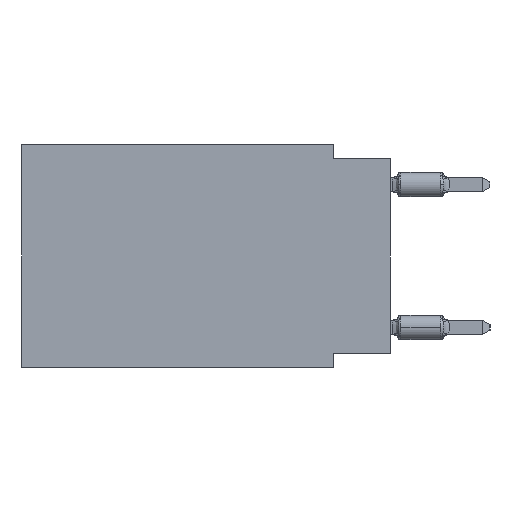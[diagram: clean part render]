
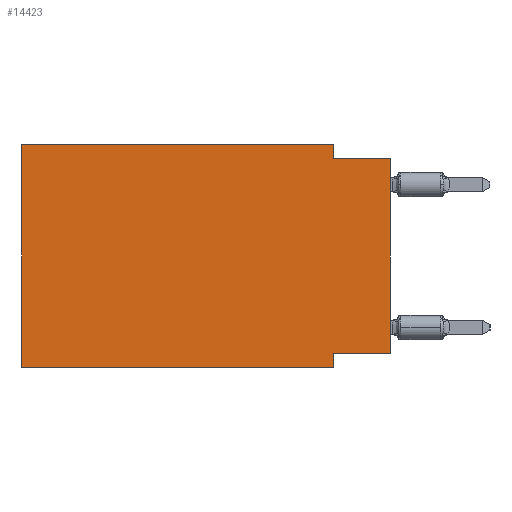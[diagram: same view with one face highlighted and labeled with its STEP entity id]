
A CAD part, left-side view. The second image highlights one B-rep face of the part: STEP entity #14423.
In plain terms, the highlighted planar face has unit normal (-1, 0, 0).
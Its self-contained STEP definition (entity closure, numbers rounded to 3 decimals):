
#656 = DIRECTION ( 'NONE',  ( 1., 0., 0. ) ) ;
#1021 = VERTEX_POINT ( 'NONE', #26408 ) ;
#1884 = DIRECTION ( 'NONE',  ( 0., -1., 0. ) ) ;
#2759 = VERTEX_POINT ( 'NONE', #11449 ) ;
#3206 = CARTESIAN_POINT ( 'NONE',  ( 0., 2.54, -9.271 ) ) ;
#4237 = ORIENTED_EDGE ( 'NONE', *, *, #25664, .F. ) ;
#4959 = VERTEX_POINT ( 'NONE', #14895 ) ;
#5066 = CARTESIAN_POINT ( 'NONE',  ( 0., 16.383, 0. ) ) ;
#6006 = DIRECTION ( 'NONE',  ( 0., 1., 0. ) ) ;
#6277 = CARTESIAN_POINT ( 'NONE',  ( 0., 2.54, -9.906 ) ) ;
#6389 = LINE ( 'NONE', #38236, #24654 ) ;
#6845 = VECTOR ( 'NONE', #6006, 1000. ) ;
#7046 = PLANE ( 'NONE',  #23246 ) ;
#7713 = DIRECTION ( 'NONE',  ( 0., 0., -1. ) ) ;
#7974 = DIRECTION ( 'NONE',  ( 0., -1., 0. ) ) ;
#8140 = VECTOR ( 'NONE', #1884, 1000. ) ;
#8549 = DIRECTION ( 'NONE',  ( 0., 0., 1. ) ) ;
#8664 = EDGE_CURVE ( 'NONE', #30264, #14222, #26211, .T. ) ;
#8927 = LINE ( 'NONE', #38065, #6845 ) ;
#10127 = VECTOR ( 'NONE', #31931, 1000. ) ;
#11442 = DIRECTION ( 'NONE',  ( 0., -1., 0. ) ) ;
#11449 = CARTESIAN_POINT ( 'NONE',  ( 0., 0., -9.271 ) ) ;
#12021 = CARTESIAN_POINT ( 'NONE',  ( 0., 16.383, -9.906 ) ) ;
#12891 = DIRECTION ( 'NONE',  ( 0., 0., -1. ) ) ;
#13048 = VECTOR ( 'NONE', #11442, 1000. ) ;
#13629 = EDGE_CURVE ( 'NONE', #31158, #14222, #31400, .T. ) ;
#13669 = VERTEX_POINT ( 'NONE', #16661 ) ;
#13751 = CARTESIAN_POINT ( 'NONE',  ( 0., 2.54, -9.906 ) ) ;
#14189 = LINE ( 'NONE', #5066, #36422 ) ;
#14222 = VERTEX_POINT ( 'NONE', #6277 ) ;
#14423 = ADVANCED_FACE ( 'NONE', ( #27827 ), #7046, .F. ) ;
#14895 = CARTESIAN_POINT ( 'NONE',  ( 0., 0., -0.635 ) ) ;
#15104 = ORIENTED_EDGE ( 'NONE', *, *, #31974, .F. ) ;
#16041 = ORIENTED_EDGE ( 'NONE', *, *, #8664, .T. ) ;
#16661 = CARTESIAN_POINT ( 'NONE',  ( 0., 2.54, 0. ) ) ;
#16776 = EDGE_LOOP ( 'NONE', ( #29357, #4237, #27468, #22241, #33281, #16041, #24893, #15104 ) ) ;
#17639 = VECTOR ( 'NONE', #7713, 1000. ) ;
#20060 = LINE ( 'NONE', #32614, #24925 ) ;
#22241 = ORIENTED_EDGE ( 'NONE', *, *, #23723, .F. ) ;
#23246 = AXIS2_PLACEMENT_3D ( 'NONE', #36187, #656, #12891 ) ;
#23496 = DIRECTION ( 'NONE',  ( 0., 0., -1. ) ) ;
#23585 = CARTESIAN_POINT ( 'NONE',  ( 0., 16.383, 0. ) ) ;
#23723 = EDGE_CURVE ( 'NONE', #34825, #13669, #14189, .T. ) ;
#23897 = EDGE_CURVE ( 'NONE', #13669, #1021, #6389, .T. ) ;
#24654 = VECTOR ( 'NONE', #23496, 1000. ) ;
#24893 = ORIENTED_EDGE ( 'NONE', *, *, #13629, .F. ) ;
#24925 = VECTOR ( 'NONE', #8549, 1000. ) ;
#25556 = CARTESIAN_POINT ( 'NONE',  ( 0., 16.383, 0. ) ) ;
#25664 = EDGE_CURVE ( 'NONE', #1021, #4959, #31381, .T. ) ;
#26025 = EDGE_CURVE ( 'NONE', #2759, #4959, #20060, .T. ) ;
#26211 = LINE ( 'NONE', #12021, #13048 ) ;
#26408 = CARTESIAN_POINT ( 'NONE',  ( 0., 2.54, -0.635 ) ) ;
#27468 = ORIENTED_EDGE ( 'NONE', *, *, #23897, .F. ) ;
#27827 = FACE_OUTER_BOUND ( 'NONE', #16776, .T. ) ;
#28470 = CARTESIAN_POINT ( 'NONE',  ( 0., 0., -0.635 ) ) ;
#29357 = ORIENTED_EDGE ( 'NONE', *, *, #26025, .T. ) ;
#30264 = VERTEX_POINT ( 'NONE', #32036 ) ;
#31158 = VERTEX_POINT ( 'NONE', #3206 ) ;
#31381 = LINE ( 'NONE', #28470, #8140 ) ;
#31400 = LINE ( 'NONE', #13751, #17639 ) ;
#31554 = LINE ( 'NONE', #25556, #10127 ) ;
#31931 = DIRECTION ( 'NONE',  ( 0., 0., 1. ) ) ;
#31974 = EDGE_CURVE ( 'NONE', #2759, #31158, #8927, .T. ) ;
#32036 = CARTESIAN_POINT ( 'NONE',  ( 0., 16.383, -9.906 ) ) ;
#32614 = CARTESIAN_POINT ( 'NONE',  ( 0., 0., 0. ) ) ;
#33281 = ORIENTED_EDGE ( 'NONE', *, *, #34654, .F. ) ;
#34654 = EDGE_CURVE ( 'NONE', #30264, #34825, #31554, .T. ) ;
#34825 = VERTEX_POINT ( 'NONE', #23585 ) ;
#36187 = CARTESIAN_POINT ( 'NONE',  ( 0., 16.383, 0. ) ) ;
#36422 = VECTOR ( 'NONE', #7974, 1000. ) ;
#38065 = CARTESIAN_POINT ( 'NONE',  ( 0., 0., -9.271 ) ) ;
#38236 = CARTESIAN_POINT ( 'NONE',  ( 0., 2.54, 0. ) ) ;
